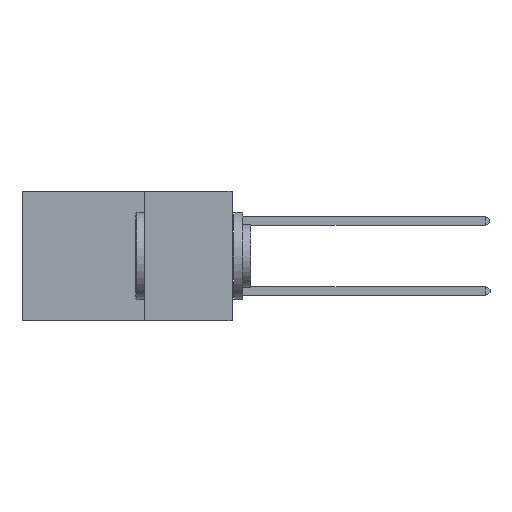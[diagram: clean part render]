
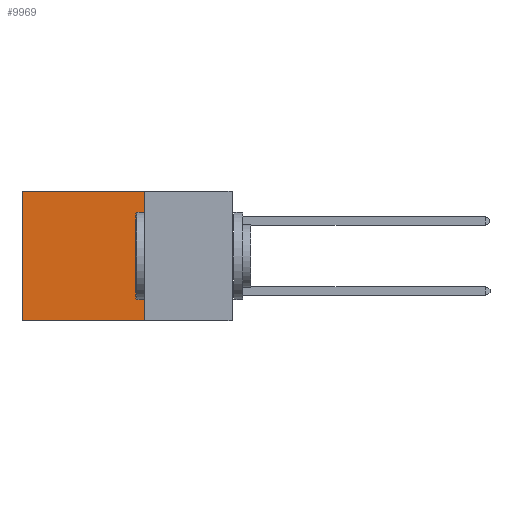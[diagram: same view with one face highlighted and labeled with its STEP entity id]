
A CAD part, left-side view. The second image highlights one B-rep face of the part: STEP entity #9969.
In plain terms, the highlighted planar face has unit normal (-1, 0, 0).
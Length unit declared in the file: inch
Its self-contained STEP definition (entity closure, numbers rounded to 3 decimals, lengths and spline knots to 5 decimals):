
#2935 = DIRECTION ( 'NONE',  ( 0., 0., -1. ) ) ;
#3156 = VERTEX_POINT ( 'NONE', #22657 ) ;
#3313 = LINE ( 'NONE', #18666, #22936 ) ;
#3842 = EDGE_LOOP ( 'NONE', ( #18168, #14818, #23066, #6072 ) ) ;
#5528 = DIRECTION ( 'NONE',  ( 0., 1., 0. ) ) ;
#6072 = ORIENTED_EDGE ( 'NONE', *, *, #22903, .T. ) ;
#6253 = DIRECTION ( 'NONE',  ( 1., 0., 0. ) ) ;
#6601 = EDGE_CURVE ( 'NONE', #12294, #8676, #3313, .T. ) ;
#7228 = CARTESIAN_POINT ( 'NONE',  ( 0.2875, 0.25, -0.37 ) ) ;
#8190 = DIRECTION ( 'NONE',  ( 0., 0., -1. ) ) ;
#8616 = LINE ( 'NONE', #14592, #11632 ) ;
#8676 = VERTEX_POINT ( 'NONE', #24136 ) ;
#9556 = EDGE_CURVE ( 'NONE', #3156, #12294, #17008, .T. ) ;
#9969 = ADVANCED_FACE ( 'NONE', ( #15498 ), #13937, .F. ) ;
#10811 = DIRECTION ( 'NONE',  ( 0., 0., -1. ) ) ;
#11297 = VECTOR ( 'NONE', #2935, 39.37008 ) ;
#11632 = VECTOR ( 'NONE', #10811, 39.37008 ) ;
#12294 = VERTEX_POINT ( 'NONE', #7228 ) ;
#12461 = CARTESIAN_POINT ( 'NONE',  ( 0.2875, 0.25, 0. ) ) ;
#13417 = VERTEX_POINT ( 'NONE', #14094 ) ;
#13937 = PLANE ( 'NONE',  #20405 ) ;
#14094 = CARTESIAN_POINT ( 'NONE',  ( 0.2875, 0.6, 0. ) ) ;
#14528 = DIRECTION ( 'NONE',  ( 0., 1., 0. ) ) ;
#14592 = CARTESIAN_POINT ( 'NONE',  ( 0.2875, 0.6, 0. ) ) ;
#14757 = LINE ( 'NONE', #20157, #24377 ) ;
#14818 = ORIENTED_EDGE ( 'NONE', *, *, #6601, .F. ) ;
#15498 = FACE_OUTER_BOUND ( 'NONE', #3842, .T. ) ;
#16183 = EDGE_CURVE ( 'NONE', #13417, #8676, #8616, .T. ) ;
#17008 = LINE ( 'NONE', #12461, #11297 ) ;
#18168 = ORIENTED_EDGE ( 'NONE', *, *, #16183, .T. ) ;
#18666 = CARTESIAN_POINT ( 'NONE',  ( 0.2875, 0.25, -0.37 ) ) ;
#19804 = CARTESIAN_POINT ( 'NONE',  ( 0.2875, 0.25, 0. ) ) ;
#20157 = CARTESIAN_POINT ( 'NONE',  ( 0.2875, 0.25, 0. ) ) ;
#20405 = AXIS2_PLACEMENT_3D ( 'NONE', #19804, #6253, #8190 ) ;
#22657 = CARTESIAN_POINT ( 'NONE',  ( 0.2875, 0.25, 0. ) ) ;
#22903 = EDGE_CURVE ( 'NONE', #3156, #13417, #14757, .T. ) ;
#22936 = VECTOR ( 'NONE', #5528, 39.37008 ) ;
#23066 = ORIENTED_EDGE ( 'NONE', *, *, #9556, .F. ) ;
#24136 = CARTESIAN_POINT ( 'NONE',  ( 0.2875, 0.6, -0.37 ) ) ;
#24377 = VECTOR ( 'NONE', #14528, 39.37008 ) ;
